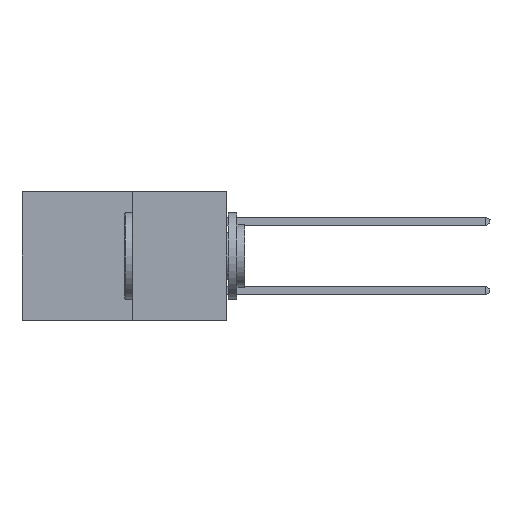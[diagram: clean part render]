
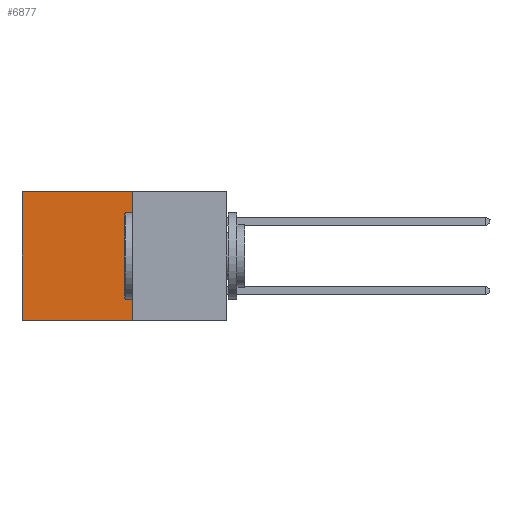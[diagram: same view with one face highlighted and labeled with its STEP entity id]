
A CAD part, left-side view. The second image highlights one B-rep face of the part: STEP entity #6877.
In plain terms, the highlighted planar face has unit normal (-1, 0, 0).
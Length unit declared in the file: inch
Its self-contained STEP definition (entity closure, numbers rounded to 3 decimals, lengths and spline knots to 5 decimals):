
#173 = EDGE_CURVE ( 'NONE', #2673, #3447, #8312, .T. ) ;
#221 = LINE ( 'NONE', #1622, #5613 ) ;
#251 = LINE ( 'NONE', #7027, #7454 ) ;
#1081 = CARTESIAN_POINT ( 'NONE',  ( 0.277, 0.59, 0. ) ) ;
#1100 = DIRECTION ( 'NONE',  ( 0., 1., 0. ) ) ;
#1225 = VECTOR ( 'NONE', #8456, 39.37008 ) ;
#1256 = FACE_OUTER_BOUND ( 'NONE', #3719, .T. ) ;
#1437 = LINE ( 'NONE', #1577, #1225 ) ;
#1577 = CARTESIAN_POINT ( 'NONE',  ( 0.277, 0.59, -0.37 ) ) ;
#1622 = CARTESIAN_POINT ( 'NONE',  ( 0.277, 0.27, -0.37 ) ) ;
#2527 = CARTESIAN_POINT ( 'NONE',  ( 0.277, 0.59, -0.37 ) ) ;
#2656 = ORIENTED_EDGE ( 'NONE', *, *, #8193, .T. ) ;
#2663 = ORIENTED_EDGE ( 'NONE', *, *, #4662, .F. ) ;
#2673 = VERTEX_POINT ( 'NONE', #7757 ) ;
#2707 = ORIENTED_EDGE ( 'NONE', *, *, #173, .F. ) ;
#2745 = ORIENTED_EDGE ( 'NONE', *, *, #3126, .T. ) ;
#3126 = EDGE_CURVE ( 'NONE', #2673, #7088, #251, .T. ) ;
#3161 = DIRECTION ( 'NONE',  ( 0., 0., -1. ) ) ;
#3165 = DIRECTION ( 'NONE',  ( 1., 0., 0. ) ) ;
#3209 = CARTESIAN_POINT ( 'NONE',  ( 0.277, 0.27, -0.37 ) ) ;
#3214 = VECTOR ( 'NONE', #4495, 39.37008 ) ;
#3369 = PLANE ( 'NONE',  #5788 ) ;
#3447 = VERTEX_POINT ( 'NONE', #4256 ) ;
#3719 = EDGE_LOOP ( 'NONE', ( #2656, #2663, #2707, #2745 ) ) ;
#4256 = CARTESIAN_POINT ( 'NONE',  ( 0.277, 0.27, -0.37 ) ) ;
#4495 = DIRECTION ( 'NONE',  ( 0., 0., -1. ) ) ;
#4662 = EDGE_CURVE ( 'NONE', #3447, #7293, #221, .T. ) ;
#5613 = VECTOR ( 'NONE', #1100, 39.37008 ) ;
#5663 = DIRECTION ( 'NONE',  ( 0., 1., 0. ) ) ;
#5788 = AXIS2_PLACEMENT_3D ( 'NONE', #3209, #3165, #3161 ) ;
#6877 = ADVANCED_FACE ( 'NONE', ( #1256 ), #3369, .F. ) ;
#7027 = CARTESIAN_POINT ( 'NONE',  ( 0.277, 0.27, 0. ) ) ;
#7088 = VERTEX_POINT ( 'NONE', #1081 ) ;
#7293 = VERTEX_POINT ( 'NONE', #2527 ) ;
#7454 = VECTOR ( 'NONE', #5663, 39.37008 ) ;
#7575 = CARTESIAN_POINT ( 'NONE',  ( 0.277, 0.27, -0.37 ) ) ;
#7757 = CARTESIAN_POINT ( 'NONE',  ( 0.277, 0.27, 0. ) ) ;
#8193 = EDGE_CURVE ( 'NONE', #7088, #7293, #1437, .T. ) ;
#8312 = LINE ( 'NONE', #7575, #3214 ) ;
#8456 = DIRECTION ( 'NONE',  ( 0., 0., -1. ) ) ;
